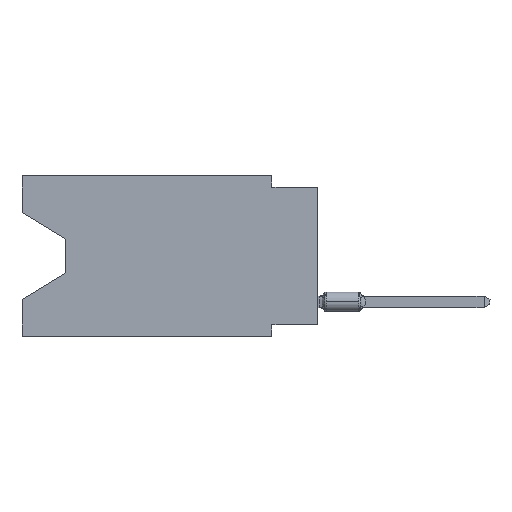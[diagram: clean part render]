
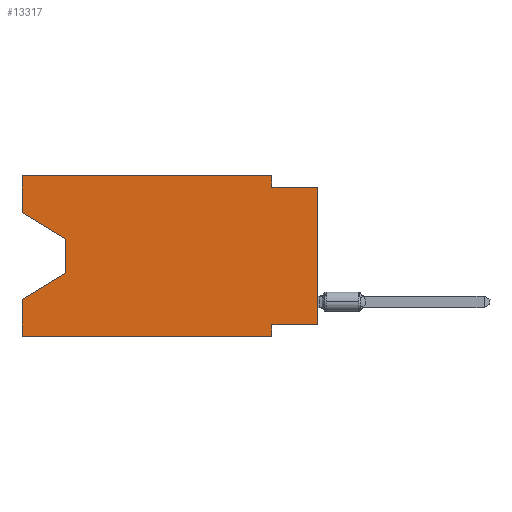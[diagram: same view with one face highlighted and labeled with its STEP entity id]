
A CAD part, left-side view. The second image highlights one B-rep face of the part: STEP entity #13317.
In plain terms, the highlighted planar face has unit normal (-1, 0, 0).
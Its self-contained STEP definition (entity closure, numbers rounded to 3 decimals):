
#965 = EDGE_LOOP ( 'NONE', ( #18478, #1787, #3749, #14218, #22556, #22089, #17073, #19660, #2322, #10934, #9117, #10762 ) ) ;
#982 = CARTESIAN_POINT ( 'NONE',  ( 0., 0., 0. ) ) ;
#1787 = ORIENTED_EDGE ( 'NONE', *, *, #21999, .T. ) ;
#1921 = VECTOR ( 'NONE', #15356, 1000. ) ;
#2322 = ORIENTED_EDGE ( 'NONE', *, *, #21681, .F. ) ;
#2614 = CARTESIAN_POINT ( 'NONE',  ( 0., 16.383, 0. ) ) ;
#3131 = DIRECTION ( 'NONE',  ( 0., -1., 0. ) ) ;
#3207 = VECTOR ( 'NONE', #6490, 1000. ) ;
#3375 = VERTEX_POINT ( 'NONE', #16364 ) ;
#3668 = VERTEX_POINT ( 'NONE', #19977 ) ;
#3748 = LINE ( 'NONE', #5335, #12805 ) ;
#3749 = ORIENTED_EDGE ( 'NONE', *, *, #4018, .T. ) ;
#4018 = EDGE_CURVE ( 'NONE', #9226, #4591, #18928, .T. ) ;
#4127 = DIRECTION ( 'NONE',  ( 0., -1., 0. ) ) ;
#4591 = VERTEX_POINT ( 'NONE', #4666 ) ;
#4666 = CARTESIAN_POINT ( 'NONE',  ( 0., 16.383, -6.852 ) ) ;
#4687 = VERTEX_POINT ( 'NONE', #23545 ) ;
#5006 = CARTESIAN_POINT ( 'NONE',  ( 0., 2.54, -0.635 ) ) ;
#5137 = VERTEX_POINT ( 'NONE', #10698 ) ;
#5335 = CARTESIAN_POINT ( 'NONE',  ( 0., 16.383, -2.038 ) ) ;
#5762 = VERTEX_POINT ( 'NONE', #16665 ) ;
#5971 = VECTOR ( 'NONE', #7798, 1000. ) ;
#6490 = DIRECTION ( 'NONE',  ( 0., 0., -1. ) ) ;
#7740 = CARTESIAN_POINT ( 'NONE',  ( 0., 16.383, -8.89 ) ) ;
#7798 = DIRECTION ( 'NONE',  ( 0., 0.855, -0.519 ) ) ;
#8278 = LINE ( 'NONE', #15665, #9400 ) ;
#8321 = EDGE_CURVE ( 'NONE', #3375, #5137, #8624, .T. ) ;
#8434 = DIRECTION ( 'NONE',  ( 0., 0., -1. ) ) ;
#8566 = CARTESIAN_POINT ( 'NONE',  ( 0., 2.54, -8.89 ) ) ;
#8624 = LINE ( 'NONE', #9103, #11720 ) ;
#8741 = DIRECTION ( 'NONE',  ( 0., 0., 1. ) ) ;
#8869 = CARTESIAN_POINT ( 'NONE',  ( 0., 16.383, -8.89 ) ) ;
#9103 = CARTESIAN_POINT ( 'NONE',  ( 0., 16.383, 0. ) ) ;
#9117 = ORIENTED_EDGE ( 'NONE', *, *, #17591, .F. ) ;
#9226 = VERTEX_POINT ( 'NONE', #13249 ) ;
#9273 = CARTESIAN_POINT ( 'NONE',  ( 0., 2.54, -8.255 ) ) ;
#9400 = VECTOR ( 'NONE', #13844, 1000. ) ;
#9771 = CARTESIAN_POINT ( 'NONE',  ( 0., 0., -8.255 ) ) ;
#9801 = CARTESIAN_POINT ( 'NONE',  ( 0., 16.383, 0. ) ) ;
#9903 = CARTESIAN_POINT ( 'NONE',  ( 0., 13.97, -3.505 ) ) ;
#10191 = VECTOR ( 'NONE', #8741, 1000. ) ;
#10227 = VECTOR ( 'NONE', #13173, 1000. ) ;
#10242 = PLANE ( 'NONE',  #22628 ) ;
#10245 = VERTEX_POINT ( 'NONE', #9903 ) ;
#10429 = LINE ( 'NONE', #17943, #16804 ) ;
#10484 = VERTEX_POINT ( 'NONE', #9273 ) ;
#10698 = CARTESIAN_POINT ( 'NONE',  ( 0., 16.383, 0. ) ) ;
#10762 = ORIENTED_EDGE ( 'NONE', *, *, #8321, .F. ) ;
#10934 = ORIENTED_EDGE ( 'NONE', *, *, #22429, .F. ) ;
#11479 = EDGE_CURVE ( 'NONE', #5762, #4687, #17812, .T. ) ;
#11720 = VECTOR ( 'NONE', #21935, 1000. ) ;
#11798 = VERTEX_POINT ( 'NONE', #8566 ) ;
#12058 = LINE ( 'NONE', #19321, #3207 ) ;
#12608 = DIRECTION ( 'NONE',  ( 0., 0., -1. ) ) ;
#12744 = VERTEX_POINT ( 'NONE', #5006 ) ;
#12755 = CARTESIAN_POINT ( 'NONE',  ( 0., 16.383, 0. ) ) ;
#12805 = VECTOR ( 'NONE', #18513, 1000. ) ;
#13173 = DIRECTION ( 'NONE',  ( 0., -1., 0. ) ) ;
#13178 = VECTOR ( 'NONE', #20139, 1000. ) ;
#13186 = LINE ( 'NONE', #9801, #19329 ) ;
#13249 = CARTESIAN_POINT ( 'NONE',  ( 0., 13.97, -5.385 ) ) ;
#13317 = ADVANCED_FACE ( 'NONE', ( #19438 ), #10242, .F. ) ;
#13844 = DIRECTION ( 'NONE',  ( 0., 0., -1. ) ) ;
#14218 = ORIENTED_EDGE ( 'NONE', *, *, #15897, .F. ) ;
#14264 = CARTESIAN_POINT ( 'NONE',  ( 0., 0., -0.635 ) ) ;
#14265 = EDGE_CURVE ( 'NONE', #10484, #11798, #10429, .T. ) ;
#14326 = EDGE_CURVE ( 'NONE', #19774, #11798, #18770, .T. ) ;
#14454 = VECTOR ( 'NONE', #3131, 1000. ) ;
#14807 = LINE ( 'NONE', #12755, #13178 ) ;
#15176 = CARTESIAN_POINT ( 'NONE',  ( 0., 13.97, -5.385 ) ) ;
#15356 = DIRECTION ( 'NONE',  ( 0., 1., 0. ) ) ;
#15665 = CARTESIAN_POINT ( 'NONE',  ( 0., 2.54, 0. ) ) ;
#15897 = EDGE_CURVE ( 'NONE', #19774, #4591, #14807, .T. ) ;
#16364 = CARTESIAN_POINT ( 'NONE',  ( 0., 16.383, -2.038 ) ) ;
#16665 = CARTESIAN_POINT ( 'NONE',  ( 0., 0., -8.255 ) ) ;
#16804 = VECTOR ( 'NONE', #12608, 1000. ) ;
#17073 = ORIENTED_EDGE ( 'NONE', *, *, #18075, .F. ) ;
#17177 = LINE ( 'NONE', #9771, #1921 ) ;
#17591 = EDGE_CURVE ( 'NONE', #5137, #3668, #13186, .T. ) ;
#17637 = DIRECTION ( 'NONE',  ( 1., 0., 0. ) ) ;
#17812 = LINE ( 'NONE', #982, #10191 ) ;
#17943 = CARTESIAN_POINT ( 'NONE',  ( 0., 2.54, -8.89 ) ) ;
#18075 = EDGE_CURVE ( 'NONE', #5762, #10484, #17177, .T. ) ;
#18478 = ORIENTED_EDGE ( 'NONE', *, *, #19095, .T. ) ;
#18513 = DIRECTION ( 'NONE',  ( 0., -0.855, -0.519 ) ) ;
#18770 = LINE ( 'NONE', #7740, #10227 ) ;
#18928 = LINE ( 'NONE', #15176, #5971 ) ;
#19095 = EDGE_CURVE ( 'NONE', #3375, #10245, #3748, .T. ) ;
#19321 = CARTESIAN_POINT ( 'NONE',  ( 0., 13.97, -3.505 ) ) ;
#19329 = VECTOR ( 'NONE', #4127, 1000. ) ;
#19438 = FACE_OUTER_BOUND ( 'NONE', #965, .T. ) ;
#19660 = ORIENTED_EDGE ( 'NONE', *, *, #11479, .T. ) ;
#19774 = VERTEX_POINT ( 'NONE', #8869 ) ;
#19977 = CARTESIAN_POINT ( 'NONE',  ( 0., 2.54, 0. ) ) ;
#20139 = DIRECTION ( 'NONE',  ( 0., 0., 1. ) ) ;
#21681 = EDGE_CURVE ( 'NONE', #12744, #4687, #23354, .T. ) ;
#21935 = DIRECTION ( 'NONE',  ( 0., 0., 1. ) ) ;
#21999 = EDGE_CURVE ( 'NONE', #10245, #9226, #12058, .T. ) ;
#22089 = ORIENTED_EDGE ( 'NONE', *, *, #14265, .F. ) ;
#22429 = EDGE_CURVE ( 'NONE', #3668, #12744, #8278, .T. ) ;
#22556 = ORIENTED_EDGE ( 'NONE', *, *, #14326, .T. ) ;
#22628 = AXIS2_PLACEMENT_3D ( 'NONE', #2614, #17637, #8434 ) ;
#23354 = LINE ( 'NONE', #14264, #14454 ) ;
#23545 = CARTESIAN_POINT ( 'NONE',  ( 0., 0., -0.635 ) ) ;
